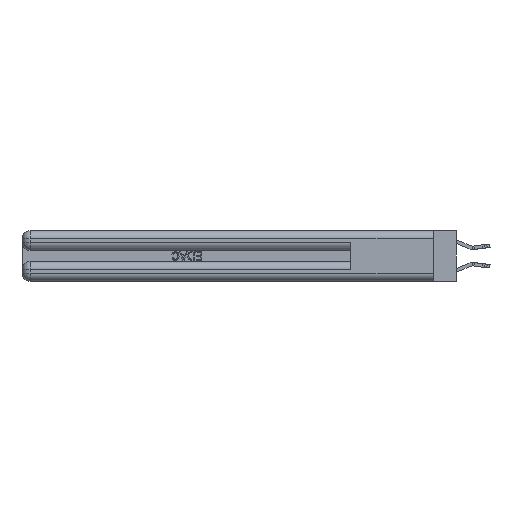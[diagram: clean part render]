
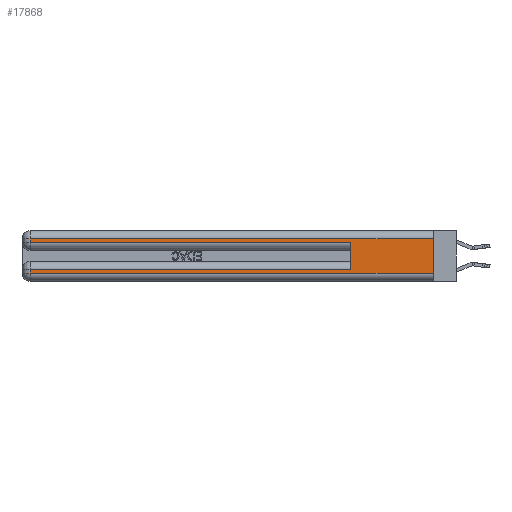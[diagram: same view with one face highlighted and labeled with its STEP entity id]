
A CAD part, left-side view. The second image highlights one B-rep face of the part: STEP entity #17868.
In plain terms, the highlighted planar face has unit normal (-1, 0, 0).
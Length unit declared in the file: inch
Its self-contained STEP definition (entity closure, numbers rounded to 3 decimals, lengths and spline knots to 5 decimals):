
#202 = ORIENTED_EDGE ( 'NONE', *, *, #25804, .T. ) ;
#259 = LINE ( 'NONE', #8707, #2186 ) ;
#739 = CARTESIAN_POINT ( 'NONE',  ( 0., 0., 0.06 ) ) ;
#1529 = ORIENTED_EDGE ( 'NONE', *, *, #19098, .T. ) ;
#1756 = CARTESIAN_POINT ( 'NONE',  ( 0., 0., 0.31 ) ) ;
#2186 = VECTOR ( 'NONE', #21476, 39.37008 ) ;
#2773 = LINE ( 'NONE', #10998, #30053 ) ;
#3366 = VECTOR ( 'NONE', #11798, 39.37008 ) ;
#3684 = DIRECTION ( 'NONE',  ( 0., 0., -1. ) ) ;
#4101 = CARTESIAN_POINT ( 'NONE',  ( 0., 0., 0.06 ) ) ;
#4495 = EDGE_CURVE ( 'NONE', #5130, #15458, #30104, .T. ) ;
#4629 = VERTEX_POINT ( 'NONE', #31267 ) ;
#4890 = ORIENTED_EDGE ( 'NONE', *, *, #26059, .T. ) ;
#5130 = VERTEX_POINT ( 'NONE', #30279 ) ;
#5635 = CARTESIAN_POINT ( 'NONE',  ( 0., 2.94, 0.06 ) ) ;
#6428 = CARTESIAN_POINT ( 'NONE',  ( 0., 0., 0.085 ) ) ;
#7062 = VERTEX_POINT ( 'NONE', #28673 ) ;
#8457 = ORIENTED_EDGE ( 'NONE', *, *, #11143, .T. ) ;
#8514 = LINE ( 'NONE', #19178, #8792 ) ;
#8602 = EDGE_CURVE ( 'NONE', #4629, #23837, #9004, .T. ) ;
#8707 = CARTESIAN_POINT ( 'NONE',  ( 0., 2.94, 0.37 ) ) ;
#8721 = AXIS2_PLACEMENT_3D ( 'NONE', #19678, #14667, #25185 ) ;
#8792 = VECTOR ( 'NONE', #3684, 39.37008 ) ;
#9004 = LINE ( 'NONE', #6428, #27297 ) ;
#9274 = DIRECTION ( 'NONE',  ( 0., 0., 1. ) ) ;
#9355 = CARTESIAN_POINT ( 'NONE',  ( 0., 2.94, 0.085 ) ) ;
#9654 = ORIENTED_EDGE ( 'NONE', *, *, #20196, .F. ) ;
#10287 = ORIENTED_EDGE ( 'NONE', *, *, #13159, .F. ) ;
#10998 = CARTESIAN_POINT ( 'NONE',  ( 0., 0., 0.37 ) ) ;
#11143 = EDGE_CURVE ( 'NONE', #23837, #32731, #8514, .T. ) ;
#11157 = DIRECTION ( 'NONE',  ( 0., 0., -1. ) ) ;
#11217 = DIRECTION ( 'NONE',  ( 0., -1., 0. ) ) ;
#11798 = DIRECTION ( 'NONE',  ( 0., -1., 0. ) ) ;
#11826 = LINE ( 'NONE', #22355, #19263 ) ;
#12216 = DIRECTION ( 'NONE',  ( 0., 1., 0. ) ) ;
#12834 = EDGE_LOOP ( 'NONE', ( #10287, #202, #1529, #32336, #9654, #31230, #8457, #4890 ) ) ;
#13159 = EDGE_CURVE ( 'NONE', #18518, #27167, #2773, .T. ) ;
#14498 = FACE_OUTER_BOUND ( 'NONE', #12834, .T. ) ;
#14667 = DIRECTION ( 'NONE',  ( 1., 0., 0. ) ) ;
#15458 = VERTEX_POINT ( 'NONE', #15960 ) ;
#15888 = LINE ( 'NONE', #739, #26600 ) ;
#15960 = CARTESIAN_POINT ( 'NONE',  ( 0., 0.6, 0.285 ) ) ;
#17197 = VECTOR ( 'NONE', #12216, 39.37008 ) ;
#17868 = ADVANCED_FACE ( 'NONE', ( #14498 ), #32941, .F. ) ;
#18518 = VERTEX_POINT ( 'NONE', #30997 ) ;
#19098 = EDGE_CURVE ( 'NONE', #7062, #5130, #259, .T. ) ;
#19178 = CARTESIAN_POINT ( 'NONE',  ( 0., 2.94, 0.37 ) ) ;
#19263 = VECTOR ( 'NONE', #9274, 39.37008 ) ;
#19678 = CARTESIAN_POINT ( 'NONE',  ( 0., 0., 0.37 ) ) ;
#20196 = EDGE_CURVE ( 'NONE', #4629, #15458, #11826, .T. ) ;
#21476 = DIRECTION ( 'NONE',  ( 0., 0., -1. ) ) ;
#22153 = CARTESIAN_POINT ( 'NONE',  ( 0., 0., 0.285 ) ) ;
#22355 = CARTESIAN_POINT ( 'NONE',  ( 0., 0.6, 0.145 ) ) ;
#23837 = VERTEX_POINT ( 'NONE', #9355 ) ;
#25185 = DIRECTION ( 'NONE',  ( 0., 0., -1. ) ) ;
#25330 = LINE ( 'NONE', #1756, #17197 ) ;
#25804 = EDGE_CURVE ( 'NONE', #18518, #7062, #25330, .T. ) ;
#26059 = EDGE_CURVE ( 'NONE', #32731, #27167, #15888, .T. ) ;
#26600 = VECTOR ( 'NONE', #11217, 39.37008 ) ;
#27087 = DIRECTION ( 'NONE',  ( 0., 1., 0. ) ) ;
#27167 = VERTEX_POINT ( 'NONE', #4101 ) ;
#27297 = VECTOR ( 'NONE', #27087, 39.37008 ) ;
#28673 = CARTESIAN_POINT ( 'NONE',  ( 0., 2.94, 0.31 ) ) ;
#30053 = VECTOR ( 'NONE', #11157, 39.37008 ) ;
#30104 = LINE ( 'NONE', #22153, #3366 ) ;
#30279 = CARTESIAN_POINT ( 'NONE',  ( 0., 2.94, 0.285 ) ) ;
#30997 = CARTESIAN_POINT ( 'NONE',  ( 0., 0., 0.31 ) ) ;
#31230 = ORIENTED_EDGE ( 'NONE', *, *, #8602, .T. ) ;
#31267 = CARTESIAN_POINT ( 'NONE',  ( 0., 0.6, 0.085 ) ) ;
#32336 = ORIENTED_EDGE ( 'NONE', *, *, #4495, .T. ) ;
#32731 = VERTEX_POINT ( 'NONE', #5635 ) ;
#32941 = PLANE ( 'NONE',  #8721 ) ;
